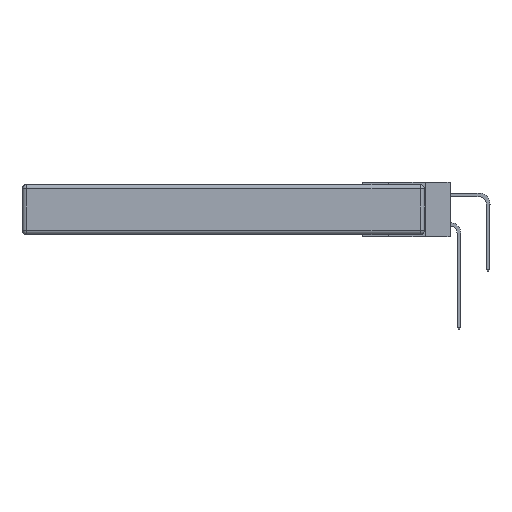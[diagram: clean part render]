
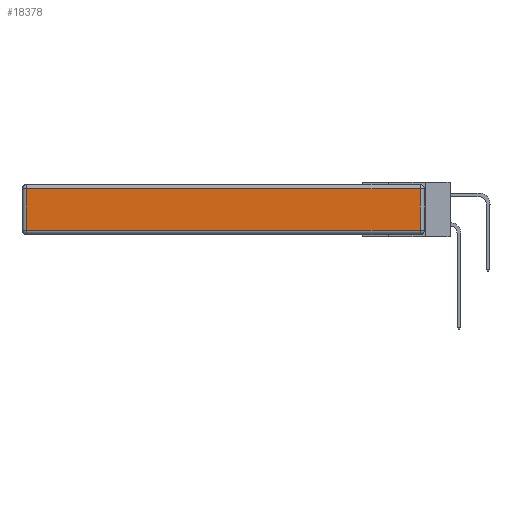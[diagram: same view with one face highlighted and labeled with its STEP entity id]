
A CAD part, left-side view. The second image highlights one B-rep face of the part: STEP entity #18378.
In plain terms, the highlighted planar face has unit normal (-1, 0, 0).
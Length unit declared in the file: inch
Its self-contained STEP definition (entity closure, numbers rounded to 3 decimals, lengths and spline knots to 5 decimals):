
#545 = CARTESIAN_POINT ( 'NONE',  ( 0., 2.75, -0.03 ) ) ;
#1388 = DIRECTION ( 'NONE',  ( 0., 0., 1. ) ) ;
#2513 = PLANE ( 'NONE',  #8575 ) ;
#2590 = CARTESIAN_POINT ( 'NONE',  ( 0., 2.72, -0.313 ) ) ;
#2976 = DIRECTION ( 'NONE',  ( 0., 1., 0. ) ) ;
#4252 = DIRECTION ( 'NONE',  ( 0., 0., -1. ) ) ;
#7434 = VECTOR ( 'NONE', #1388, 39.37008 ) ;
#7439 = DIRECTION ( 'NONE',  ( 0., -1., 0. ) ) ;
#8250 = CARTESIAN_POINT ( 'NONE',  ( 0., 0.03, -0.343 ) ) ;
#8457 = VECTOR ( 'NONE', #7439, 39.37008 ) ;
#8575 = AXIS2_PLACEMENT_3D ( 'NONE', #24278, #21988, #26712 ) ;
#9680 = CARTESIAN_POINT ( 'NONE',  ( 0., 0., -0.313 ) ) ;
#10091 = CARTESIAN_POINT ( 'NONE',  ( 0., 0.03, -0.313 ) ) ;
#10211 = EDGE_CURVE ( 'NONE', #12124, #12270, #28941, .T. ) ;
#10817 = EDGE_LOOP ( 'NONE', ( #19288, #16443, #17815, #27437 ) ) ;
#11023 = VECTOR ( 'NONE', #4252, 39.37008 ) ;
#12124 = VERTEX_POINT ( 'NONE', #13425 ) ;
#12270 = VERTEX_POINT ( 'NONE', #17845 ) ;
#13425 = CARTESIAN_POINT ( 'NONE',  ( 0., 0.03, -0.03 ) ) ;
#14944 = VERTEX_POINT ( 'NONE', #10091 ) ;
#15285 = EDGE_CURVE ( 'NONE', #14944, #12124, #21167, .T. ) ;
#15321 = VECTOR ( 'NONE', #2976, 39.37008 ) ;
#15338 = LINE ( 'NONE', #9680, #8457 ) ;
#16443 = ORIENTED_EDGE ( 'NONE', *, *, #15285, .T. ) ;
#17470 = LINE ( 'NONE', #30894, #11023 ) ;
#17815 = ORIENTED_EDGE ( 'NONE', *, *, #10211, .T. ) ;
#17845 = CARTESIAN_POINT ( 'NONE',  ( 0., 2.72, -0.03 ) ) ;
#18378 = ADVANCED_FACE ( 'NONE', ( #29991 ), #2513, .T. ) ;
#19288 = ORIENTED_EDGE ( 'NONE', *, *, #26447, .T. ) ;
#21167 = LINE ( 'NONE', #8250, #7434 ) ;
#21988 = DIRECTION ( 'NONE',  ( -1., 0., 0. ) ) ;
#22151 = VERTEX_POINT ( 'NONE', #2590 ) ;
#24278 = CARTESIAN_POINT ( 'NONE',  ( 0., 0., -0.343 ) ) ;
#26447 = EDGE_CURVE ( 'NONE', #22151, #14944, #15338, .T. ) ;
#26712 = DIRECTION ( 'NONE',  ( 0., 0., 1. ) ) ;
#27437 = ORIENTED_EDGE ( 'NONE', *, *, #28602, .T. ) ;
#28602 = EDGE_CURVE ( 'NONE', #12270, #22151, #17470, .T. ) ;
#28941 = LINE ( 'NONE', #545, #15321 ) ;
#29991 = FACE_OUTER_BOUND ( 'NONE', #10817, .T. ) ;
#30894 = CARTESIAN_POINT ( 'NONE',  ( 0., 2.72, -0.343 ) ) ;
